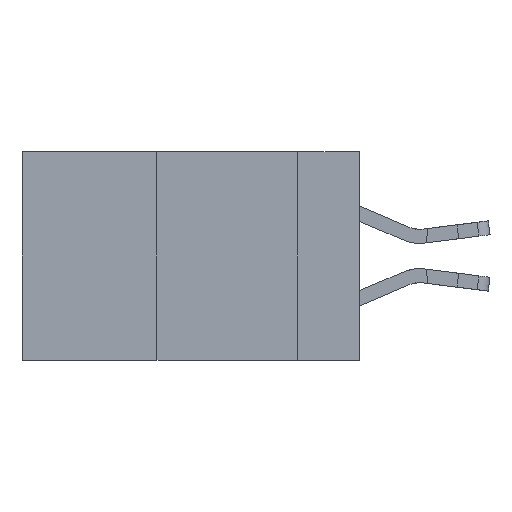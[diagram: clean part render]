
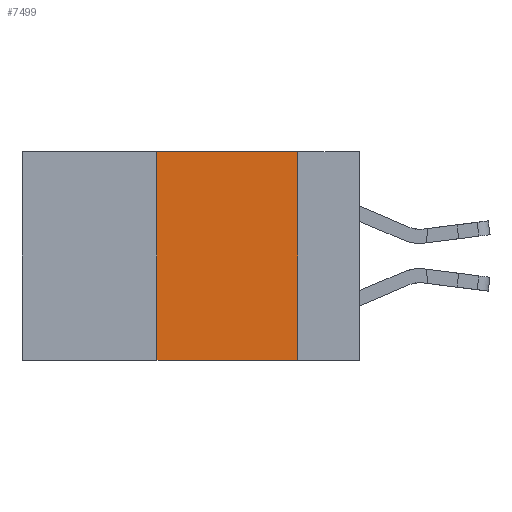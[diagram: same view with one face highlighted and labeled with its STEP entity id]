
A CAD part, left-side view. The second image highlights one B-rep face of the part: STEP entity #7499.
In plain terms, the highlighted planar face has unit normal (-1, 0, 0).
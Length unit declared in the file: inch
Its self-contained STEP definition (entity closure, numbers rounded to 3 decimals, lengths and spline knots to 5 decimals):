
#896 = CARTESIAN_POINT ( 'NONE',  ( 0., 0.11, 0. ) ) ;
#972 = DIRECTION ( 'NONE',  ( 0., 0., -1. ) ) ;
#1662 = VECTOR ( 'NONE', #1910, 39.37008 ) ;
#1910 = DIRECTION ( 'NONE',  ( 0., -1., 0. ) ) ;
#2688 = LINE ( 'NONE', #21333, #19480 ) ;
#5189 = ORIENTED_EDGE ( 'NONE', *, *, #17074, .T. ) ;
#5807 = EDGE_CURVE ( 'NONE', #6412, #20384, #6153, .T. ) ;
#5961 = VERTEX_POINT ( 'NONE', #20643 ) ;
#6153 = LINE ( 'NONE', #18630, #1662 ) ;
#6222 = EDGE_CURVE ( 'NONE', #18259, #6412, #2688, .T. ) ;
#6340 = LINE ( 'NONE', #896, #10334 ) ;
#6412 = VERTEX_POINT ( 'NONE', #10195 ) ;
#7499 = ADVANCED_FACE ( 'NONE', ( #16592 ), #19669, .F. ) ;
#7701 = CARTESIAN_POINT ( 'NONE',  ( 0., 0.11, 0. ) ) ;
#7996 = CARTESIAN_POINT ( 'NONE',  ( 0., 0.6, 0. ) ) ;
#9709 = DIRECTION ( 'NONE',  ( 1., 0., 0. ) ) ;
#10195 = CARTESIAN_POINT ( 'NONE',  ( 0., 0.36, 0. ) ) ;
#10266 = ORIENTED_EDGE ( 'NONE', *, *, #6222, .F. ) ;
#10334 = VECTOR ( 'NONE', #972, 39.37008 ) ;
#10410 = EDGE_CURVE ( 'NONE', #20384, #5961, #6340, .T. ) ;
#10966 = CARTESIAN_POINT ( 'NONE',  ( 0., 0.6, -0.37 ) ) ;
#12579 = DIRECTION ( 'NONE',  ( 0., -1., 0. ) ) ;
#12690 = CARTESIAN_POINT ( 'NONE',  ( 0., 0.36, -0.37 ) ) ;
#13049 = DIRECTION ( 'NONE',  ( 0., 0., 1. ) ) ;
#14571 = EDGE_LOOP ( 'NONE', ( #17872, #18496, #10266, #5189 ) ) ;
#16592 = FACE_OUTER_BOUND ( 'NONE', #14571, .T. ) ;
#17074 = EDGE_CURVE ( 'NONE', #18259, #5961, #19227, .T. ) ;
#17437 = AXIS2_PLACEMENT_3D ( 'NONE', #7996, #9709, #21296 ) ;
#17872 = ORIENTED_EDGE ( 'NONE', *, *, #10410, .F. ) ;
#18259 = VERTEX_POINT ( 'NONE', #12690 ) ;
#18496 = ORIENTED_EDGE ( 'NONE', *, *, #5807, .F. ) ;
#18630 = CARTESIAN_POINT ( 'NONE',  ( 0., 0.6, 0. ) ) ;
#18696 = VECTOR ( 'NONE', #12579, 39.37008 ) ;
#19227 = LINE ( 'NONE', #10966, #18696 ) ;
#19480 = VECTOR ( 'NONE', #13049, 39.37008 ) ;
#19669 = PLANE ( 'NONE',  #17437 ) ;
#20384 = VERTEX_POINT ( 'NONE', #7701 ) ;
#20643 = CARTESIAN_POINT ( 'NONE',  ( 0., 0.11, -0.37 ) ) ;
#21296 = DIRECTION ( 'NONE',  ( 0., 0., -1. ) ) ;
#21333 = CARTESIAN_POINT ( 'NONE',  ( 0., 0.36, 0. ) ) ;
